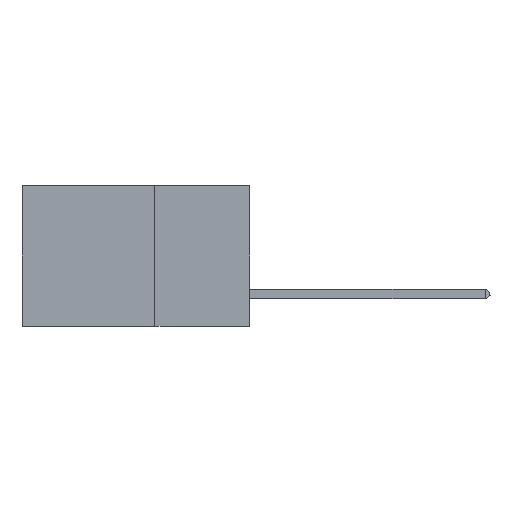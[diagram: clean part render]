
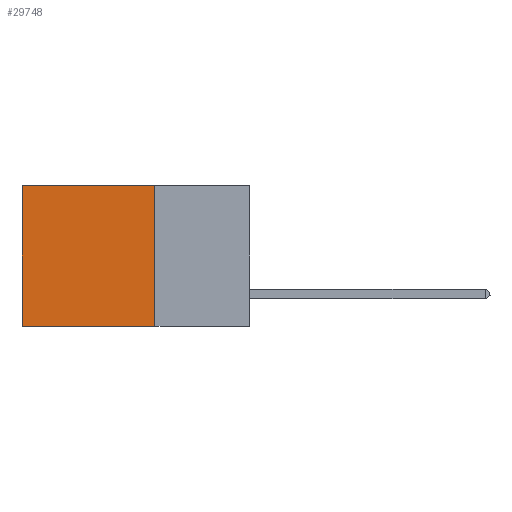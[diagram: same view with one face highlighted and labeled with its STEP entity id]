
A CAD part, left-side view. The second image highlights one B-rep face of the part: STEP entity #29748.
In plain terms, the highlighted planar face has unit normal (-1, 0, 0).
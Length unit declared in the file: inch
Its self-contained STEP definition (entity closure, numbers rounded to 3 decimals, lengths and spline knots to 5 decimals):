
#89 = DIRECTION ( 'NONE',  ( 1., 0., 0. ) ) ;
#120 = ORIENTED_EDGE ( 'NONE', *, *, #23975, .T. ) ;
#399 = DIRECTION ( 'NONE',  ( 0., 0., -1. ) ) ;
#406 = CARTESIAN_POINT ( 'NONE',  ( 0.2875, 0.25, 0. ) ) ;
#700 = DIRECTION ( 'NONE',  ( 0., 1., 0. ) ) ;
#1271 = CARTESIAN_POINT ( 'NONE',  ( 0.2875, 0.25, 0. ) ) ;
#3225 = VECTOR ( 'NONE', #24672, 39.37008 ) ;
#6010 = EDGE_CURVE ( 'NONE', #28781, #24663, #15310, .T. ) ;
#7782 = DIRECTION ( 'NONE',  ( 0., 1., 0. ) ) ;
#8334 = LINE ( 'NONE', #46528, #3225 ) ;
#10203 = EDGE_CURVE ( 'NONE', #16607, #17352, #19993, .T. ) ;
#11383 = DIRECTION ( 'NONE',  ( 0., 0., -1. ) ) ;
#14274 = CARTESIAN_POINT ( 'NONE',  ( 0.2875, 0.25, 0. ) ) ;
#14736 = FACE_OUTER_BOUND ( 'NONE', #28698, .T. ) ;
#15310 = LINE ( 'NONE', #22558, #31735 ) ;
#16607 = VERTEX_POINT ( 'NONE', #1271 ) ;
#17352 = VERTEX_POINT ( 'NONE', #38921 ) ;
#19993 = LINE ( 'NONE', #22492, #42598 ) ;
#22492 = CARTESIAN_POINT ( 'NONE',  ( 0.2875, 0.25, 0. ) ) ;
#22558 = CARTESIAN_POINT ( 'NONE',  ( 0.2875, 0.25, -0.37 ) ) ;
#23546 = ORIENTED_EDGE ( 'NONE', *, *, #6010, .F. ) ;
#23975 = EDGE_CURVE ( 'NONE', #17352, #24663, #8334, .T. ) ;
#24663 = VERTEX_POINT ( 'NONE', #34180 ) ;
#24672 = DIRECTION ( 'NONE',  ( 0., 0., -1. ) ) ;
#26997 = AXIS2_PLACEMENT_3D ( 'NONE', #14274, #89, #399 ) ;
#28698 = EDGE_LOOP ( 'NONE', ( #120, #23546, #36090, #32991 ) ) ;
#28781 = VERTEX_POINT ( 'NONE', #38376 ) ;
#29748 = ADVANCED_FACE ( 'NONE', ( #14736 ), #32795, .F. ) ;
#31735 = VECTOR ( 'NONE', #7782, 39.37008 ) ;
#32795 = PLANE ( 'NONE',  #26997 ) ;
#32991 = ORIENTED_EDGE ( 'NONE', *, *, #10203, .T. ) ;
#34180 = CARTESIAN_POINT ( 'NONE',  ( 0.2875, 0.6, -0.37 ) ) ;
#35725 = LINE ( 'NONE', #406, #39124 ) ;
#35846 = EDGE_CURVE ( 'NONE', #16607, #28781, #35725, .T. ) ;
#36090 = ORIENTED_EDGE ( 'NONE', *, *, #35846, .F. ) ;
#38376 = CARTESIAN_POINT ( 'NONE',  ( 0.2875, 0.25, -0.37 ) ) ;
#38921 = CARTESIAN_POINT ( 'NONE',  ( 0.2875, 0.6, 0. ) ) ;
#39124 = VECTOR ( 'NONE', #11383, 39.37008 ) ;
#42598 = VECTOR ( 'NONE', #700, 39.37008 ) ;
#46528 = CARTESIAN_POINT ( 'NONE',  ( 0.2875, 0.6, 0. ) ) ;
